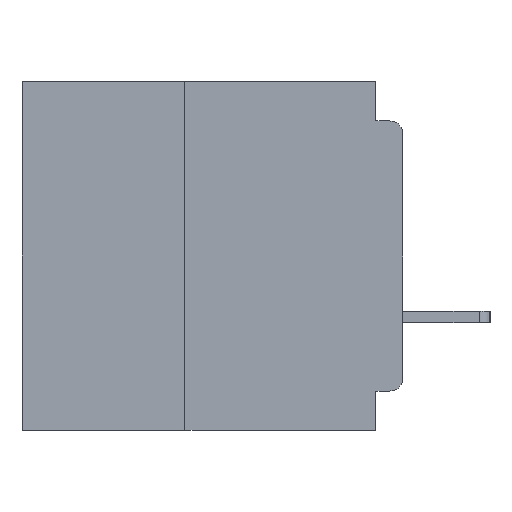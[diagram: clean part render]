
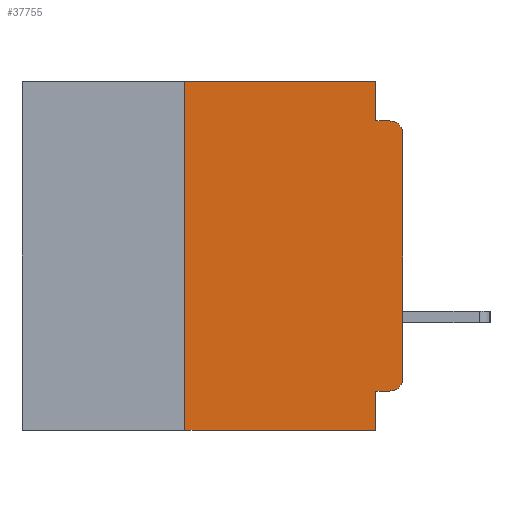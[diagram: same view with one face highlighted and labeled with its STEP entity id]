
A CAD part, left-side view. The second image highlights one B-rep face of the part: STEP entity #37755.
In plain terms, the highlighted planar face has unit normal (-1, 0, 0).
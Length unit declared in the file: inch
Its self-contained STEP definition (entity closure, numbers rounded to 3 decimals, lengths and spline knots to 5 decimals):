
#71 = CIRCLE ( 'NONE', #19073, 0.015 ) ;
#538 = VECTOR ( 'NONE', #8569, 39.37008 ) ;
#1913 = VERTEX_POINT ( 'NONE', #16484 ) ;
#1965 = EDGE_CURVE ( 'NONE', #38391, #32251, #4332, .T. ) ;
#2771 = DIRECTION ( 'NONE',  ( 0., 0., -1. ) ) ;
#3628 = EDGE_CURVE ( 'NONE', #1913, #25044, #15926, .T. ) ;
#4089 = ORIENTED_EDGE ( 'NONE', *, *, #28590, .F. ) ;
#4332 = CIRCLE ( 'NONE', #17578, 0.015 ) ;
#4890 = DIRECTION ( 'NONE',  ( 0., -1., 0. ) ) ;
#5860 = ORIENTED_EDGE ( 'NONE', *, *, #3628, .F. ) ;
#6236 = CARTESIAN_POINT ( 'NONE',  ( 0., 0.437, 0. ) ) ;
#7340 = CARTESIAN_POINT ( 'NONE',  ( 0., 0., -0.045 ) ) ;
#7444 = VECTOR ( 'NONE', #19896, 39.37008 ) ;
#7532 = FACE_OUTER_BOUND ( 'NONE', #31107, .T. ) ;
#8082 = CARTESIAN_POINT ( 'NONE',  ( 0., 0., 0. ) ) ;
#8094 = VERTEX_POINT ( 'NONE', #43049 ) ;
#8445 = ORIENTED_EDGE ( 'NONE', *, *, #41129, .F. ) ;
#8569 = DIRECTION ( 'NONE',  ( 0., 1., 0. ) ) ;
#9060 = VECTOR ( 'NONE', #34563, 39.37008 ) ;
#9944 = PLANE ( 'NONE',  #10767 ) ;
#10767 = AXIS2_PLACEMENT_3D ( 'NONE', #6236, #21288, #47513 ) ;
#10999 = EDGE_CURVE ( 'NONE', #32251, #40638, #42377, .T. ) ;
#11937 = EDGE_CURVE ( 'NONE', #40638, #8094, #71, .T. ) ;
#12761 = DIRECTION ( 'NONE',  ( 0., 0., -1. ) ) ;
#13581 = VECTOR ( 'NONE', #4890, 39.37008 ) ;
#13613 = ORIENTED_EDGE ( 'NONE', *, *, #11937, .T. ) ;
#14401 = ORIENTED_EDGE ( 'NONE', *, *, #10999, .T. ) ;
#14579 = VECTOR ( 'NONE', #14827, 39.37008 ) ;
#14643 = CARTESIAN_POINT ( 'NONE',  ( 0., 0.015, -0.355 ) ) ;
#14827 = DIRECTION ( 'NONE',  ( 0., -1., 0. ) ) ;
#15926 = LINE ( 'NONE', #27347, #13581 ) ;
#16484 = CARTESIAN_POINT ( 'NONE',  ( 0., 0.25, 0. ) ) ;
#16813 = DIRECTION ( 'NONE',  ( -1., 0., 0. ) ) ;
#17397 = CARTESIAN_POINT ( 'NONE',  ( 0., 0.031, -0.355 ) ) ;
#17578 = AXIS2_PLACEMENT_3D ( 'NONE', #39319, #16813, #43056 ) ;
#18337 = VECTOR ( 'NONE', #12761, 39.37008 ) ;
#19073 = AXIS2_PLACEMENT_3D ( 'NONE', #47647, #25215, #2771 ) ;
#19508 = EDGE_CURVE ( 'NONE', #38391, #29243, #29282, .T. ) ;
#19896 = DIRECTION ( 'NONE',  ( 0., 0., 1. ) ) ;
#20240 = LINE ( 'NONE', #26979, #9060 ) ;
#21288 = DIRECTION ( 'NONE',  ( 1., 0., 0. ) ) ;
#23150 = DIRECTION ( 'NONE',  ( 0., 0., 1. ) ) ;
#23556 = VERTEX_POINT ( 'NONE', #39376 ) ;
#24689 = LINE ( 'NONE', #47567, #43447 ) ;
#25018 = ORIENTED_EDGE ( 'NONE', *, *, #19508, .F. ) ;
#25044 = VERTEX_POINT ( 'NONE', #41367 ) ;
#25215 = DIRECTION ( 'NONE',  ( -1., 0., 0. ) ) ;
#26979 = CARTESIAN_POINT ( 'NONE',  ( 0., 0.031, -0.4 ) ) ;
#27347 = CARTESIAN_POINT ( 'NONE',  ( 0., 0.437, 0. ) ) ;
#27777 = CARTESIAN_POINT ( 'NONE',  ( 0., 0., -0.06 ) ) ;
#28357 = LINE ( 'NONE', #35325, #18337 ) ;
#28582 = LINE ( 'NONE', #42356, #7444 ) ;
#28590 = EDGE_CURVE ( 'NONE', #29243, #38347, #20240, .T. ) ;
#29243 = VERTEX_POINT ( 'NONE', #17397 ) ;
#29282 = LINE ( 'NONE', #31074, #538 ) ;
#29296 = CARTESIAN_POINT ( 'NONE',  ( 0., 0.031, -0.4 ) ) ;
#29349 = CARTESIAN_POINT ( 'NONE',  ( 0., 0., -0.34 ) ) ;
#29986 = CARTESIAN_POINT ( 'NONE',  ( 0., 0.25, -0.4 ) ) ;
#30060 = VERTEX_POINT ( 'NONE', #29986 ) ;
#31074 = CARTESIAN_POINT ( 'NONE',  ( 0., 0., -0.355 ) ) ;
#31090 = EDGE_CURVE ( 'NONE', #30060, #38347, #24689, .T. ) ;
#31107 = EDGE_LOOP ( 'NONE', ( #14401, #13613, #45124, #8445, #5860, #37446, #35541, #4089, #25018, #43952 ) ) ;
#32251 = VERTEX_POINT ( 'NONE', #29349 ) ;
#32434 = VECTOR ( 'NONE', #23150, 39.37008 ) ;
#32672 = DIRECTION ( 'NONE',  ( 0., -1., 0. ) ) ;
#34563 = DIRECTION ( 'NONE',  ( 0., 0., -1. ) ) ;
#35325 = CARTESIAN_POINT ( 'NONE',  ( 0., 0.031, 0. ) ) ;
#35541 = ORIENTED_EDGE ( 'NONE', *, *, #31090, .T. ) ;
#37146 = EDGE_CURVE ( 'NONE', #23556, #8094, #44529, .T. ) ;
#37446 = ORIENTED_EDGE ( 'NONE', *, *, #38631, .F. ) ;
#37755 = ADVANCED_FACE ( 'NONE', ( #7532 ), #9944, .F. ) ;
#38347 = VERTEX_POINT ( 'NONE', #29296 ) ;
#38391 = VERTEX_POINT ( 'NONE', #14643 ) ;
#38631 = EDGE_CURVE ( 'NONE', #30060, #1913, #28582, .T. ) ;
#39319 = CARTESIAN_POINT ( 'NONE',  ( 0., 0.015, -0.34 ) ) ;
#39376 = CARTESIAN_POINT ( 'NONE',  ( 0., 0.031, -0.045 ) ) ;
#40638 = VERTEX_POINT ( 'NONE', #27777 ) ;
#41129 = EDGE_CURVE ( 'NONE', #25044, #23556, #28357, .T. ) ;
#41367 = CARTESIAN_POINT ( 'NONE',  ( 0., 0.031, 0. ) ) ;
#42356 = CARTESIAN_POINT ( 'NONE',  ( 0., 0.25, -0.4 ) ) ;
#42377 = LINE ( 'NONE', #8082, #32434 ) ;
#43049 = CARTESIAN_POINT ( 'NONE',  ( 0., 0.015, -0.045 ) ) ;
#43056 = DIRECTION ( 'NONE',  ( 0., 0., -1. ) ) ;
#43447 = VECTOR ( 'NONE', #32672, 39.37008 ) ;
#43952 = ORIENTED_EDGE ( 'NONE', *, *, #1965, .T. ) ;
#44529 = LINE ( 'NONE', #7340, #14579 ) ;
#45124 = ORIENTED_EDGE ( 'NONE', *, *, #37146, .F. ) ;
#47513 = DIRECTION ( 'NONE',  ( 0., 0., -1. ) ) ;
#47567 = CARTESIAN_POINT ( 'NONE',  ( 0., 0.437, -0.4 ) ) ;
#47647 = CARTESIAN_POINT ( 'NONE',  ( 0., 0.015, -0.06 ) ) ;
